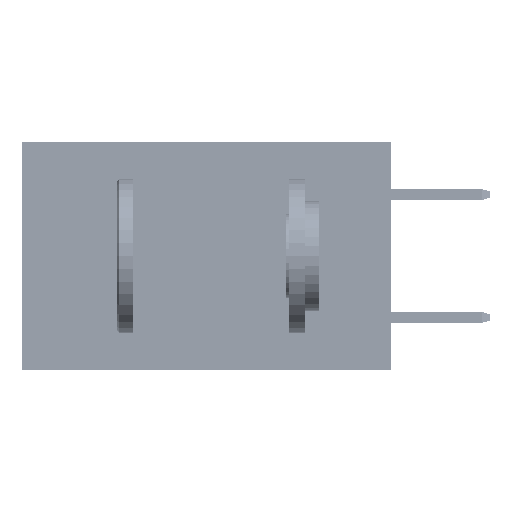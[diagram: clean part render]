
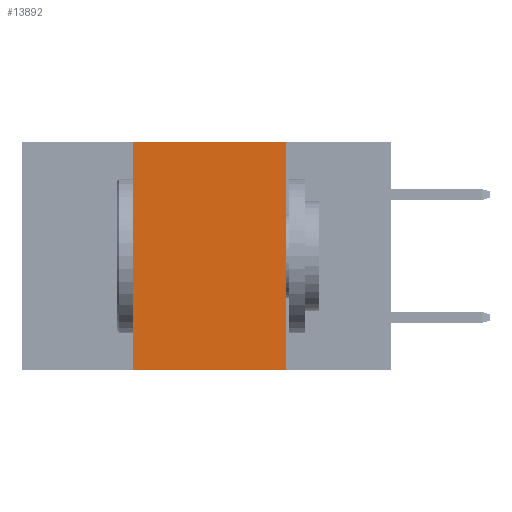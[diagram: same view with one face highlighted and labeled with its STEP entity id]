
A CAD part, left-side view. The second image highlights one B-rep face of the part: STEP entity #13892.
In plain terms, the highlighted planar face has unit normal (-1, 0, 0).
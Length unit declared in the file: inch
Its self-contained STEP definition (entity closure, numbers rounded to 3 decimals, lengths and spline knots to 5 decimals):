
#23 = DIRECTION ( 'NONE',  ( 0., -1., 0. ) ) ;
#5330 = LINE ( 'NONE', #5463, #43385 ) ;
#5463 = CARTESIAN_POINT ( 'NONE',  ( 0., 0.42, 0. ) ) ;
#6080 = DIRECTION ( 'NONE',  ( 0., 0., -1. ) ) ;
#6255 = CARTESIAN_POINT ( 'NONE',  ( 0., 0.6, 0. ) ) ;
#7581 = VERTEX_POINT ( 'NONE', #36009 ) ;
#9416 = AXIS2_PLACEMENT_3D ( 'NONE', #6255, #22160, #6080 ) ;
#11133 = LINE ( 'NONE', #38108, #22633 ) ;
#13892 = ADVANCED_FACE ( 'NONE', ( #32143 ), #29239, .F. ) ;
#18138 = EDGE_CURVE ( 'NONE', #42660, #22955, #47470, .T. ) ;
#18571 = DIRECTION ( 'NONE',  ( 0., 0., -1. ) ) ;
#18860 = EDGE_CURVE ( 'NONE', #7581, #22955, #11133, .T. ) ;
#19014 = CARTESIAN_POINT ( 'NONE',  ( 0., 0.6, 0. ) ) ;
#20258 = LINE ( 'NONE', #19014, #40820 ) ;
#21549 = ORIENTED_EDGE ( 'NONE', *, *, #18860, .T. ) ;
#21809 = ORIENTED_EDGE ( 'NONE', *, *, #38806, .F. ) ;
#22152 = ORIENTED_EDGE ( 'NONE', *, *, #37302, .F. ) ;
#22160 = DIRECTION ( 'NONE',  ( 1., 0., 0. ) ) ;
#22633 = VECTOR ( 'NONE', #23, 39.37008 ) ;
#22681 = VECTOR ( 'NONE', #18571, 39.37008 ) ;
#22955 = VERTEX_POINT ( 'NONE', #33413 ) ;
#25197 = VERTEX_POINT ( 'NONE', #37237 ) ;
#25207 = CARTESIAN_POINT ( 'NONE',  ( 0., 0.17, 0. ) ) ;
#29239 = PLANE ( 'NONE',  #9416 ) ;
#32015 = EDGE_LOOP ( 'NONE', ( #43492, #21809, #22152, #21549 ) ) ;
#32143 = FACE_OUTER_BOUND ( 'NONE', #32015, .T. ) ;
#33413 = CARTESIAN_POINT ( 'NONE',  ( 0., 0.17, -0.37 ) ) ;
#34711 = DIRECTION ( 'NONE',  ( 0., -1., 0. ) ) ;
#36009 = CARTESIAN_POINT ( 'NONE',  ( 0., 0.42, -0.37 ) ) ;
#36374 = DIRECTION ( 'NONE',  ( 0., 0., 1. ) ) ;
#37237 = CARTESIAN_POINT ( 'NONE',  ( 0., 0.42, 0. ) ) ;
#37302 = EDGE_CURVE ( 'NONE', #7581, #25197, #5330, .T. ) ;
#38108 = CARTESIAN_POINT ( 'NONE',  ( 0., 0.6, -0.37 ) ) ;
#38806 = EDGE_CURVE ( 'NONE', #25197, #42660, #20258, .T. ) ;
#40820 = VECTOR ( 'NONE', #34711, 39.37008 ) ;
#42379 = CARTESIAN_POINT ( 'NONE',  ( 0., 0.17, 0. ) ) ;
#42660 = VERTEX_POINT ( 'NONE', #25207 ) ;
#43385 = VECTOR ( 'NONE', #36374, 39.37008 ) ;
#43492 = ORIENTED_EDGE ( 'NONE', *, *, #18138, .F. ) ;
#47470 = LINE ( 'NONE', #42379, #22681 ) ;
